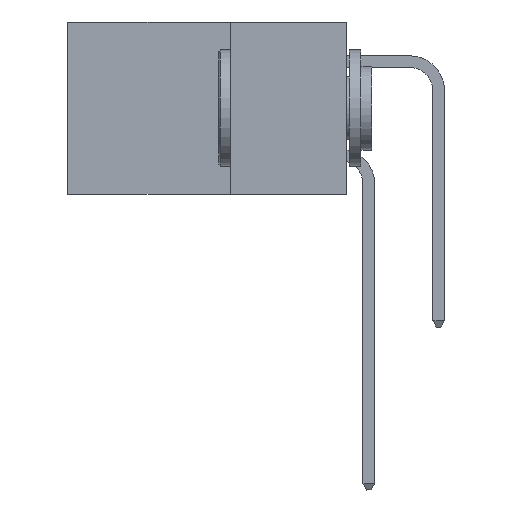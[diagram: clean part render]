
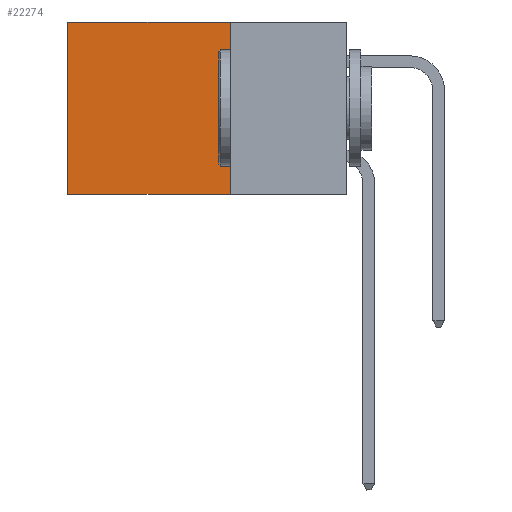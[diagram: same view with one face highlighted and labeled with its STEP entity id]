
A CAD part, left-side view. The second image highlights one B-rep face of the part: STEP entity #22274.
In plain terms, the highlighted planar face has unit normal (-1, 0, 0).
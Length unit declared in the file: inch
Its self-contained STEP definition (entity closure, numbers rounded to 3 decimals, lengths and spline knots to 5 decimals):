
#31 = VECTOR ( 'NONE', #3558, 39.37008 ) ;
#2361 = VERTEX_POINT ( 'NONE', #20346 ) ;
#3481 = DIRECTION ( 'NONE',  ( 1., 0., 0. ) ) ;
#3558 = DIRECTION ( 'NONE',  ( 0., 0., -1. ) ) ;
#5251 = CARTESIAN_POINT ( 'NONE',  ( 0.2875, 0.6, 0. ) ) ;
#6013 = EDGE_CURVE ( 'NONE', #21277, #34562, #35523, .T. ) ;
#6109 = CARTESIAN_POINT ( 'NONE',  ( 0.2875, 0.25, -0.37 ) ) ;
#6416 = ORIENTED_EDGE ( 'NONE', *, *, #33286, .F. ) ;
#6755 = DIRECTION ( 'NONE',  ( 0., 0., -1. ) ) ;
#6865 = VECTOR ( 'NONE', #8940, 39.37008 ) ;
#7951 = VECTOR ( 'NONE', #29885, 39.37008 ) ;
#8142 = CARTESIAN_POINT ( 'NONE',  ( 0.2875, 0.25, 0. ) ) ;
#8162 = EDGE_CURVE ( 'NONE', #34562, #2361, #18810, .T. ) ;
#8940 = DIRECTION ( 'NONE',  ( 0., 1., 0. ) ) ;
#10444 = CARTESIAN_POINT ( 'NONE',  ( 0.2875, 0.25, -0.37 ) ) ;
#12440 = ORIENTED_EDGE ( 'NONE', *, *, #25701, .F. ) ;
#13253 = DIRECTION ( 'NONE',  ( 0., 1., 0. ) ) ;
#14613 = PLANE ( 'NONE',  #32942 ) ;
#18810 = LINE ( 'NONE', #5251, #7951 ) ;
#19852 = CARTESIAN_POINT ( 'NONE',  ( 0.2875, 0.25, 0. ) ) ;
#20346 = CARTESIAN_POINT ( 'NONE',  ( 0.2875, 0.6, -0.37 ) ) ;
#20732 = ORIENTED_EDGE ( 'NONE', *, *, #6013, .T. ) ;
#21277 = VERTEX_POINT ( 'NONE', #8142 ) ;
#21337 = VECTOR ( 'NONE', #13253, 39.37008 ) ;
#22274 = ADVANCED_FACE ( 'NONE', ( #25432 ), #14613, .F. ) ;
#23360 = CARTESIAN_POINT ( 'NONE',  ( 0.2875, 0.25, 0. ) ) ;
#25244 = VERTEX_POINT ( 'NONE', #6109 ) ;
#25432 = FACE_OUTER_BOUND ( 'NONE', #35539, .T. ) ;
#25701 = EDGE_CURVE ( 'NONE', #25244, #2361, #28268, .T. ) ;
#27340 = CARTESIAN_POINT ( 'NONE',  ( 0.2875, 0.6, 0. ) ) ;
#28268 = LINE ( 'NONE', #10444, #21337 ) ;
#28923 = CARTESIAN_POINT ( 'NONE',  ( 0.2875, 0.25, 0. ) ) ;
#29885 = DIRECTION ( 'NONE',  ( 0., 0., -1. ) ) ;
#32038 = ORIENTED_EDGE ( 'NONE', *, *, #8162, .T. ) ;
#32942 = AXIS2_PLACEMENT_3D ( 'NONE', #23360, #3481, #6755 ) ;
#33286 = EDGE_CURVE ( 'NONE', #21277, #25244, #34333, .T. ) ;
#34333 = LINE ( 'NONE', #28923, #31 ) ;
#34562 = VERTEX_POINT ( 'NONE', #27340 ) ;
#35523 = LINE ( 'NONE', #19852, #6865 ) ;
#35539 = EDGE_LOOP ( 'NONE', ( #32038, #12440, #6416, #20732 ) ) ;
